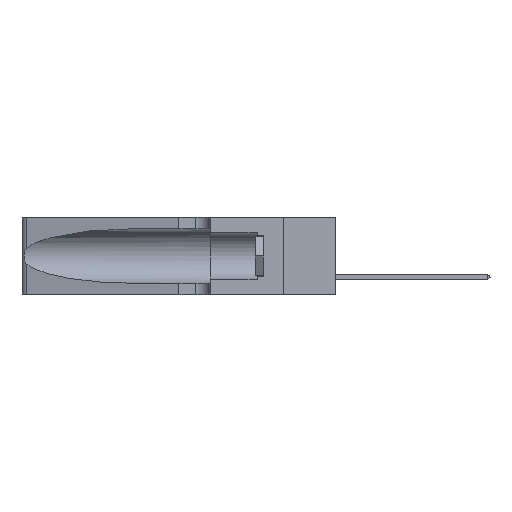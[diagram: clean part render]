
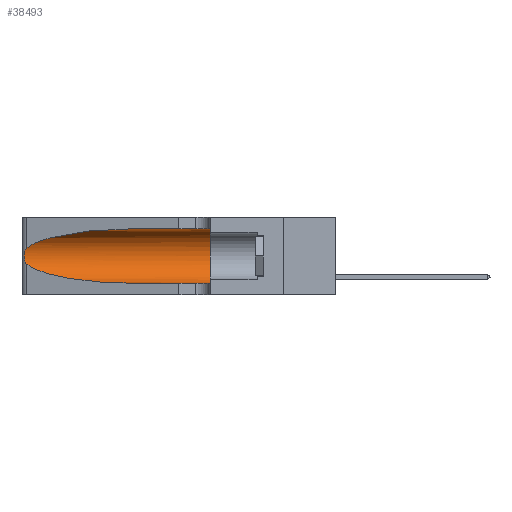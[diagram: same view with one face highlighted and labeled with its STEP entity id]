
A CAD part, left-side view. The second image highlights one B-rep face of the part: STEP entity #38493.
In plain terms, the highlighted cylindrical face has radius 3.308 mm (diameter 6.617 mm), a partial arc.
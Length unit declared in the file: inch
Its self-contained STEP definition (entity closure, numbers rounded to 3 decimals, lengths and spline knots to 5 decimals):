
#577 = CARTESIAN_POINT ( 'NONE',  ( 0.1305, 1.61858, 0.31525 ) ) ;
#1636 = CARTESIAN_POINT ( 'NONE',  ( 0.26075, 1.23896, 0.19203 ) ) ;
#3353 = VERTEX_POINT ( 'NONE', #23952 ) ;
#5192 = CARTESIAN_POINT ( 'NONE',  ( 0.25856, 1.23593, 0.16098 ) ) ;
#5574 = CARTESIAN_POINT ( 'NONE',  ( 0.25487, 1.22718, 0.22369 ) ) ;
#5880 = CARTESIAN_POINT ( 'NONE',  ( 0.25787, 1.23484, 0.2124 ) ) ;
#7801 = VERTEX_POINT ( 'NONE', #47793 ) ;
#8012 = VERTEX_POINT ( 'NONE', #5574 ) ;
#8437 = CARTESIAN_POINT ( 'NONE',  ( 0.18966, 0.96281, 0.05475 ) ) ;
#8609 = ORIENTED_EDGE ( 'NONE', *, *, #21204, .T. ) ;
#9759 = CARTESIAN_POINT ( 'NONE',  ( 0.26075, 1.23896, 0.178 ) ) ;
#10186 = CARTESIAN_POINT ( 'NONE',  ( 0.1305, 0.72297, 0.05475 ) ) ;
#10200 = VERTEX_POINT ( 'NONE', #30613 ) ;
#11253 = DIRECTION ( 'NONE',  ( 0., -1., 0. ) ) ;
#13274 = CARTESIAN_POINT ( 'NONE',  ( 0.25639, 1.23184, 0.21858 ) ) ;
#13449 = CARTESIAN_POINT ( 'NONE',  ( 0.25487, 1.22718, 0.22369 ) ) ;
#13746 = ORIENTED_EDGE ( 'NONE', *, *, #41670, .F. ) ;
#13978 = CARTESIAN_POINT ( 'NONE',  ( 0.25555, 1.22994, 0.2215 ) ) ;
#14140 = CIRCLE ( 'NONE', #51362, 0.13025 ) ;
#15539 = CARTESIAN_POINT ( 'NONE',  ( 0.1305, 0.35, 0.31525 ) ) ;
#17713 = CARTESIAN_POINT ( 'NONE',  ( 0.26017, 1.23833, 0.17102 ) ) ;
#17847 = AXIS2_PLACEMENT_3D ( 'NONE', #19548, #11253, #39747 ) ;
#17882 = CARTESIAN_POINT ( 'NONE',  ( 0.25487, 1.22718, 0.14631 ) ) ;
#19104 = ORIENTED_EDGE ( 'NONE', *, *, #34522, .T. ) ;
#19314 = CARTESIAN_POINT ( 'NONE',  ( 0.25487, 1.22718, 0.22369 ) ) ;
#19548 = CARTESIAN_POINT ( 'NONE',  ( 0.1305, 1.61858, 0.185 ) ) ;
#20590 = CARTESIAN_POINT ( 'NONE',  ( 0.1305, 0.72297, 0.05475 ) ) ;
#21204 = EDGE_CURVE ( 'NONE', #8012, #7801, #37053, .T. ) ;
#22072 = EDGE_CURVE ( 'NONE', #3353, #8012, #47924, .T. ) ;
#23021 = CARTESIAN_POINT ( 'NONE',  ( 0.2373, 1.15595, 0.28018 ) ) ;
#23952 = CARTESIAN_POINT ( 'NONE',  ( 0.1305, 0.72297, 0.31525 ) ) ;
#26088 = LINE ( 'NONE', #45215, #38040 ) ;
#27969 = DIRECTION ( 'NONE',  ( 0., 1., 0. ) ) ;
#29477 = ORIENTED_EDGE ( 'NONE', *, *, #38041, .T. ) ;
#29676 = CARTESIAN_POINT ( 'NONE',  ( 0.25639, 1.23186, 0.15144 ) ) ;
#30613 = CARTESIAN_POINT ( 'NONE',  ( 0.1305, 0.35, 0.05475 ) ) ;
#31544 = ORIENTED_EDGE ( 'NONE', *, *, #46292, .F. ) ;
#31812 = CARTESIAN_POINT ( 'NONE',  ( 0.18966, 0.96281, 0.31525 ) ) ;
#32129 = VERTEX_POINT ( 'NONE', #15539 ) ;
#33156 = DIRECTION ( 'NONE',  ( 0., -1., 0. ) ) ;
#34234 = LINE ( 'NONE', #577, #47393 ) ;
#34522 = EDGE_CURVE ( 'NONE', #7801, #40615, #50841, .T. ) ;
#36798 = CARTESIAN_POINT ( 'NONE',  ( 0.25487, 1.22718, 0.14631 ) ) ;
#37053 = B_SPLINE_CURVE_WITH_KNOTS ( 'NONE', 3,
 ( #13449, #13978, #13274, #5880, #46136, #37750, #1636, #9759, #17713, #5192, #41788, #29676, #41605, #17882 ),
 .UNSPECIFIED., .F., .F.,
 ( 4, 2, 2, 2, 2, 2, 4 ),
 ( 0., 0.00027, 0.00053, 0.00107, 0.0016, 0.00187, 0.00214 ),
 .UNSPECIFIED. ) ;
#37750 = CARTESIAN_POINT ( 'NONE',  ( 0.26018, 1.23835, 0.19895 ) ) ;
#38040 = VECTOR ( 'NONE', #41063, 39.37008 ) ;
#38041 = EDGE_CURVE ( 'NONE', #40615, #10200, #26088, .T. ) ;
#38365 = CYLINDRICAL_SURFACE ( 'NONE', #17847, 0.13025 ) ;
#38493 = ADVANCED_FACE ( 'NONE', ( #43969 ), #38365, .F. ) ;
#39747 = DIRECTION ( 'NONE',  ( 0., 0., -1. ) ) ;
#40615 = VERTEX_POINT ( 'NONE', #10186 ) ;
#40619 = CARTESIAN_POINT ( 'NONE',  ( 0.1305, 0.35, 0.185 ) ) ;
#40643 = CARTESIAN_POINT ( 'NONE',  ( 0.2373, 1.15595, 0.08982 ) ) ;
#41063 = DIRECTION ( 'NONE',  ( 0., -1., 0. ) ) ;
#41605 = CARTESIAN_POINT ( 'NONE',  ( 0.25555, 1.22993, 0.14849 ) ) ;
#41670 = EDGE_CURVE ( 'NONE', #3353, #32129, #34234, .T. ) ;
#41788 = CARTESIAN_POINT ( 'NONE',  ( 0.25789, 1.23486, 0.15765 ) ) ;
#43969 = FACE_OUTER_BOUND ( 'NONE', #51808, .T. ) ;
#44628 = DIRECTION ( 'NONE',  ( 0., 0., 1. ) ) ;
#45215 = CARTESIAN_POINT ( 'NONE',  ( 0.1305, 1.61858, 0.05475 ) ) ;
#45705 = ORIENTED_EDGE ( 'NONE', *, *, #22072, .T. ) ;
#46136 = CARTESIAN_POINT ( 'NONE',  ( 0.25854, 1.2359, 0.20912 ) ) ;
#46292 = EDGE_CURVE ( 'NONE', #32129, #10200, #14140, .T. ) ;
#47213 = CARTESIAN_POINT ( 'NONE',  ( 0.1305, 0.72297, 0.31525 ) ) ;
#47393 = VECTOR ( 'NONE', #33156, 39.37008 ) ;
#47793 = CARTESIAN_POINT ( 'NONE',  ( 0.25487, 1.22718, 0.14631 ) ) ;
#47924 =( BOUNDED_CURVE ( )  B_SPLINE_CURVE ( 3, ( #47213, #31812, #23021, #19314 ),
 .UNSPECIFIED., .F., .F. ) 
 B_SPLINE_CURVE_WITH_KNOTS ( ( 4, 4 ),
 ( 1.5708, 2.84003 ),
 .UNSPECIFIED. ) 
 CURVE ( )  GEOMETRIC_REPRESENTATION_ITEM ( )  RATIONAL_B_SPLINE_CURVE ( ( 1., 0.87, 0.87, 1. ) ) 
 REPRESENTATION_ITEM ( '' )  );
#50841 =( BOUNDED_CURVE ( )  B_SPLINE_CURVE ( 3, ( #36798, #40643, #8437, #20590 ),
 .UNSPECIFIED., .F., .F. ) 
 B_SPLINE_CURVE_WITH_KNOTS ( ( 4, 4 ),
 ( 3.44316, 4.71239 ),
 .UNSPECIFIED. ) 
 CURVE ( )  GEOMETRIC_REPRESENTATION_ITEM ( )  RATIONAL_B_SPLINE_CURVE ( ( 1., 0.87, 0.87, 1. ) ) 
 REPRESENTATION_ITEM ( '' )  );
#51362 = AXIS2_PLACEMENT_3D ( 'NONE', #40619, #27969, #44628 ) ;
#51808 = EDGE_LOOP ( 'NONE', ( #45705, #8609, #19104, #29477, #31544, #13746 ) ) ;
